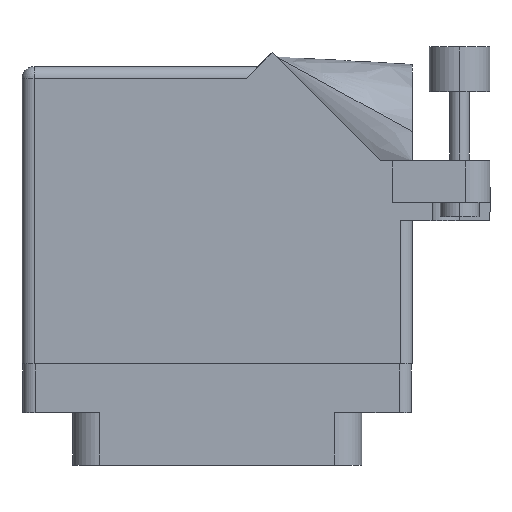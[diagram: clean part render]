
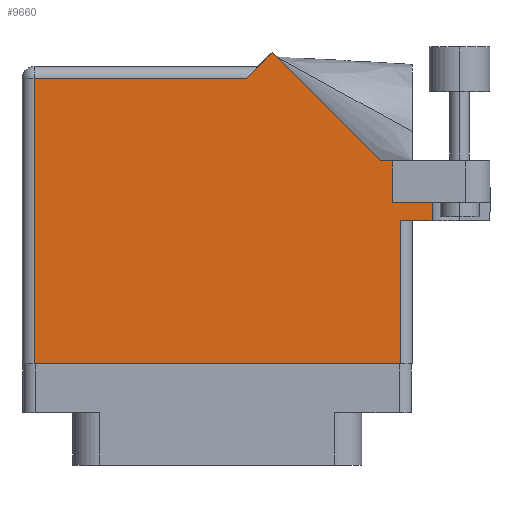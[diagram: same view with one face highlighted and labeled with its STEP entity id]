
A CAD part, front view. The second image highlights one B-rep face of the part: STEP entity #9660.
In plain terms, the highlighted face is planar.
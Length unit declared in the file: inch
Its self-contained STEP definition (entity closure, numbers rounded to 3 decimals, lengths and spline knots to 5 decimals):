
#1324 = DIRECTION ( 'NONE',  ( -0.707, 0.707, 0. ) ) ;
#1336 = ORIENTED_EDGE ( 'NONE', *, *, #25861, .T. ) ;
#1393 = DIRECTION ( 'NONE',  ( 0., -1., 0. ) ) ;
#2865 = EDGE_CURVE ( 'NONE', #11695, #3677, #10674, .T. ) ;
#3370 = DIRECTION ( 'NONE',  ( 0., 1., 0. ) ) ;
#3398 = LINE ( 'NONE', #34349, #17059 ) ;
#3538 = CARTESIAN_POINT ( 'NONE',  ( -0.943, 1.368, 0.455 ) ) ;
#3677 = VERTEX_POINT ( 'NONE', #3538 ) ;
#3949 = CARTESIAN_POINT ( 'NONE',  ( 0.83942, 0.944, 0.455 ) ) ;
#4318 = CARTESIAN_POINT ( 'NONE',  ( -1.005, -0.1, 0.455 ) ) ;
#4462 = VECTOR ( 'NONE', #1324, 39.37008 ) ;
#4579 = LINE ( 'NONE', #17085, #6539 ) ;
#5000 = VERTEX_POINT ( 'NONE', #5817 ) ;
#5817 = CARTESIAN_POINT ( 'NONE',  ( -0.943, -0.1, 0.455 ) ) ;
#6539 = VECTOR ( 'NONE', #26428, 39.37008 ) ;
#6879 = VERTEX_POINT ( 'NONE', #29053 ) ;
#7280 = LINE ( 'NONE', #20219, #23920 ) ;
#7952 = EDGE_CURVE ( 'NONE', #8731, #29906, #13026, .T. ) ;
#8731 = VERTEX_POINT ( 'NONE', #24017 ) ;
#8916 = AXIS2_PLACEMENT_3D ( 'NONE', #27240, #17508, #30233 ) ;
#9007 = CARTESIAN_POINT ( 'NONE',  ( 1.1065, 0.731, 0.455 ) ) ;
#9660 = ADVANCED_FACE ( 'NONE', ( #36337 ), #29970, .F. ) ;
#9923 = ORIENTED_EDGE ( 'NONE', *, *, #35369, .T. ) ;
#10081 = EDGE_CURVE ( 'NONE', #30325, #10290, #14776, .T. ) ;
#10290 = VERTEX_POINT ( 'NONE', #11962 ) ;
#10674 = LINE ( 'NONE', #26921, #13618 ) ;
#11087 = CARTESIAN_POINT ( 'NONE',  ( 0.905, 0.944, 0.455 ) ) ;
#11115 = CARTESIAN_POINT ( 'NONE',  ( 0.905, 0.731, 0.455 ) ) ;
#11372 = CARTESIAN_POINT ( 'NONE',  ( 0.15, 1.368, 0.455 ) ) ;
#11695 = VERTEX_POINT ( 'NONE', #11372 ) ;
#11962 = CARTESIAN_POINT ( 'NONE',  ( 1.1065, 0.637, 0.455 ) ) ;
#13026 = LINE ( 'NONE', #14544, #28245 ) ;
#13618 = VECTOR ( 'NONE', #33299, 39.37008 ) ;
#14244 = DIRECTION ( 'NONE',  ( 1., 0., 0. ) ) ;
#14544 = CARTESIAN_POINT ( 'NONE',  ( 0.905, 0.731, 0.455 ) ) ;
#14776 = LINE ( 'NONE', #19813, #33839 ) ;
#14996 = ORIENTED_EDGE ( 'NONE', *, *, #39324, .T. ) ;
#15017 = ORIENTED_EDGE ( 'NONE', *, *, #28932, .T. ) ;
#15317 = LINE ( 'NONE', #39032, #21763 ) ;
#17017 = VECTOR ( 'NONE', #17050, 39.37008 ) ;
#17050 = DIRECTION ( 'NONE',  ( -1., 0., 0. ) ) ;
#17059 = VECTOR ( 'NONE', #3370, 39.37008 ) ;
#17085 = CARTESIAN_POINT ( 'NONE',  ( -0.943, -0.1, 0.455 ) ) ;
#17508 = DIRECTION ( 'NONE',  ( 0., 0., -1. ) ) ;
#19241 = EDGE_CURVE ( 'NONE', #24352, #30946, #30840, .T. ) ;
#19391 = DIRECTION ( 'NONE',  ( 1., 0., 0. ) ) ;
#19605 = CARTESIAN_POINT ( 'NONE',  ( 0.83942, 0.944, 0.455 ) ) ;
#19813 = CARTESIAN_POINT ( 'NONE',  ( 1.005, 0.637, 0.455 ) ) ;
#20219 = CARTESIAN_POINT ( 'NONE',  ( 0.212, 1.43, 0.455 ) ) ;
#20291 = EDGE_CURVE ( 'NONE', #30946, #11695, #7280, .T. ) ;
#20309 = DIRECTION ( 'NONE',  ( 0., 1., 0. ) ) ;
#21380 = VERTEX_POINT ( 'NONE', #11087 ) ;
#21439 = VECTOR ( 'NONE', #14244, 39.37008 ) ;
#21763 = VECTOR ( 'NONE', #1393, 39.37008 ) ;
#21809 = EDGE_CURVE ( 'NONE', #29906, #10290, #15317, .T. ) ;
#21991 = EDGE_LOOP ( 'NONE', ( #15017, #27919, #39510, #24652, #28520, #14996, #1336, #25132, #38516, #31450, #9923 ) ) ;
#23627 = DIRECTION ( 'NONE',  ( 1., 0., 0. ) ) ;
#23720 = CARTESIAN_POINT ( 'NONE',  ( 0.943, 0.637, 0.455 ) ) ;
#23869 = LINE ( 'NONE', #4318, #21439 ) ;
#23920 = VECTOR ( 'NONE', #32901, 39.37008 ) ;
#24017 = CARTESIAN_POINT ( 'NONE',  ( 0.905, 0.731, 0.455 ) ) ;
#24352 = VERTEX_POINT ( 'NONE', #3949 ) ;
#24652 = ORIENTED_EDGE ( 'NONE', *, *, #21809, .F. ) ;
#25132 = ORIENTED_EDGE ( 'NONE', *, *, #19241, .T. ) ;
#25861 = EDGE_CURVE ( 'NONE', #21380, #24352, #37035, .T. ) ;
#26428 = DIRECTION ( 'NONE',  ( 0., -1., 0. ) ) ;
#26830 = VECTOR ( 'NONE', #20309, 39.37008 ) ;
#26921 = CARTESIAN_POINT ( 'NONE',  ( -1.005, 1.368, 0.455 ) ) ;
#27240 = CARTESIAN_POINT ( 'NONE',  ( -1.005, 1.43, 0.455 ) ) ;
#27804 = LINE ( 'NONE', #11115, #26830 ) ;
#27919 = ORIENTED_EDGE ( 'NONE', *, *, #34137, .T. ) ;
#28245 = VECTOR ( 'NONE', #23627, 39.37008 ) ;
#28520 = ORIENTED_EDGE ( 'NONE', *, *, #7952, .F. ) ;
#28932 = EDGE_CURVE ( 'NONE', #5000, #6879, #23869, .T. ) ;
#29053 = CARTESIAN_POINT ( 'NONE',  ( 0.943, -0.1, 0.455 ) ) ;
#29388 = CARTESIAN_POINT ( 'NONE',  ( 1.405, 0.944, 0.455 ) ) ;
#29906 = VERTEX_POINT ( 'NONE', #9007 ) ;
#29970 = PLANE ( 'NONE',  #8916 ) ;
#30233 = DIRECTION ( 'NONE',  ( -1., 0., 0. ) ) ;
#30325 = VERTEX_POINT ( 'NONE', #23720 ) ;
#30840 = LINE ( 'NONE', #19605, #4462 ) ;
#30946 = VERTEX_POINT ( 'NONE', #31826 ) ;
#31450 = ORIENTED_EDGE ( 'NONE', *, *, #2865, .T. ) ;
#31826 = CARTESIAN_POINT ( 'NONE',  ( 0.28271, 1.50071, 0.455 ) ) ;
#32901 = DIRECTION ( 'NONE',  ( -0.707, -0.707, 0. ) ) ;
#33299 = DIRECTION ( 'NONE',  ( -1., 0., 0. ) ) ;
#33839 = VECTOR ( 'NONE', #19391, 39.37008 ) ;
#34137 = EDGE_CURVE ( 'NONE', #6879, #30325, #3398, .T. ) ;
#34349 = CARTESIAN_POINT ( 'NONE',  ( 0.943, 0.637, 0.455 ) ) ;
#35369 = EDGE_CURVE ( 'NONE', #3677, #5000, #4579, .T. ) ;
#36337 = FACE_OUTER_BOUND ( 'NONE', #21991, .T. ) ;
#37035 = LINE ( 'NONE', #29388, #17017 ) ;
#38516 = ORIENTED_EDGE ( 'NONE', *, *, #20291, .T. ) ;
#39032 = CARTESIAN_POINT ( 'NONE',  ( 1.1065, 1.06177, 0.455 ) ) ;
#39324 = EDGE_CURVE ( 'NONE', #8731, #21380, #27804, .T. ) ;
#39510 = ORIENTED_EDGE ( 'NONE', *, *, #10081, .T. ) ;
